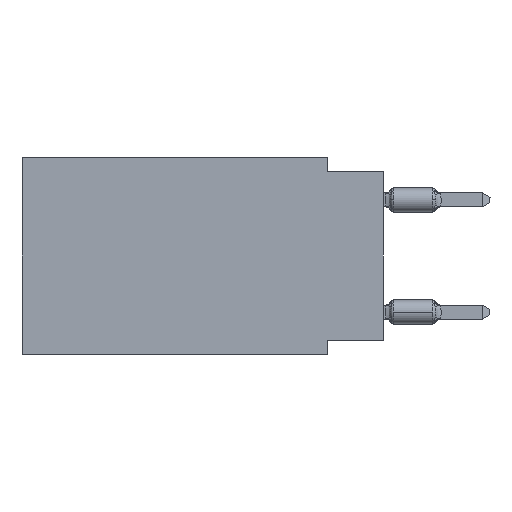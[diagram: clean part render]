
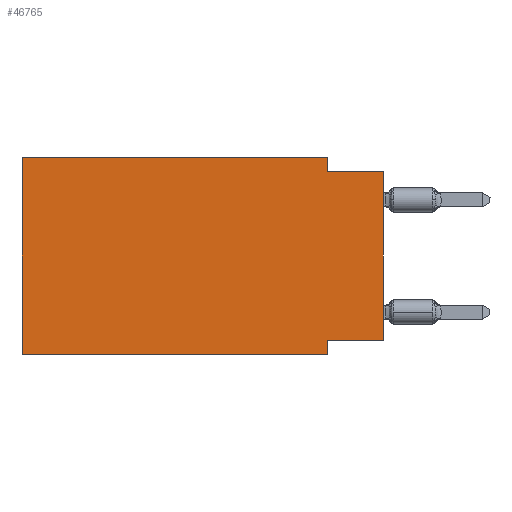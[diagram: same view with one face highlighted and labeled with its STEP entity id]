
A CAD part, left-side view. The second image highlights one B-rep face of the part: STEP entity #46765.
In plain terms, the highlighted planar face has unit normal (-1, 0, 0).
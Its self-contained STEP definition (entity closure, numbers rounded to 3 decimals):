
#680 = CARTESIAN_POINT ( 'NONE',  ( 0., 0., -8.255 ) ) ;
#1125 = EDGE_CURVE ( 'NONE', #8151, #5050, #22016, .T. ) ;
#1750 = LINE ( 'NONE', #14236, #53486 ) ;
#1891 = CARTESIAN_POINT ( 'NONE',  ( 0., 2.54, -8.255 ) ) ;
#3690 = CARTESIAN_POINT ( 'NONE',  ( 0., 2.54, -8.89 ) ) ;
#4180 = ORIENTED_EDGE ( 'NONE', *, *, #1125, .T. ) ;
#5050 = VERTEX_POINT ( 'NONE', #16949 ) ;
#5253 = DIRECTION ( 'NONE',  ( 0., -1., 0. ) ) ;
#7419 = PLANE ( 'NONE',  #43557 ) ;
#8151 = VERTEX_POINT ( 'NONE', #37151 ) ;
#10588 = VECTOR ( 'NONE', #20522, 1000. ) ;
#11175 = DIRECTION ( 'NONE',  ( 0., 0., -1. ) ) ;
#12456 = VECTOR ( 'NONE', #52749, 1000. ) ;
#13107 = VERTEX_POINT ( 'NONE', #30770 ) ;
#13301 = VECTOR ( 'NONE', #11175, 1000. ) ;
#13368 = ORIENTED_EDGE ( 'NONE', *, *, #31567, .F. ) ;
#14236 = CARTESIAN_POINT ( 'NONE',  ( 0., 0., -0.635 ) ) ;
#14434 = VECTOR ( 'NONE', #21892, 1000. ) ;
#15368 = EDGE_CURVE ( 'NONE', #13107, #5050, #1750, .T. ) ;
#16724 = VERTEX_POINT ( 'NONE', #43879 ) ;
#16949 = CARTESIAN_POINT ( 'NONE',  ( 0., 0., -0.635 ) ) ;
#19416 = EDGE_CURVE ( 'NONE', #8151, #51653, #33802, .T. ) ;
#20129 = EDGE_CURVE ( 'NONE', #25563, #13107, #27487, .T. ) ;
#20522 = DIRECTION ( 'NONE',  ( 0., 1., 0. ) ) ;
#21892 = DIRECTION ( 'NONE',  ( 0., -1., 0. ) ) ;
#22016 = LINE ( 'NONE', #34785, #38747 ) ;
#24004 = CARTESIAN_POINT ( 'NONE',  ( 0., 16.383, 0. ) ) ;
#24983 = ORIENTED_EDGE ( 'NONE', *, *, #49805, .T. ) ;
#25563 = VERTEX_POINT ( 'NONE', #28155 ) ;
#25857 = VERTEX_POINT ( 'NONE', #33251 ) ;
#25971 = CARTESIAN_POINT ( 'NONE',  ( 0., 16.383, 0. ) ) ;
#27487 = LINE ( 'NONE', #32343, #13301 ) ;
#28155 = CARTESIAN_POINT ( 'NONE',  ( 0., 2.54, 0. ) ) ;
#28202 = LINE ( 'NONE', #32821, #12456 ) ;
#30053 = LINE ( 'NONE', #25971, #14434 ) ;
#30770 = CARTESIAN_POINT ( 'NONE',  ( 0., 2.54, -0.635 ) ) ;
#31567 = EDGE_CURVE ( 'NONE', #45171, #25857, #28202, .T. ) ;
#32343 = CARTESIAN_POINT ( 'NONE',  ( 0., 2.54, 0. ) ) ;
#32821 = CARTESIAN_POINT ( 'NONE',  ( 0., 16.383, 0. ) ) ;
#32971 = CARTESIAN_POINT ( 'NONE',  ( 0., 16.383, -8.89 ) ) ;
#33251 = CARTESIAN_POINT ( 'NONE',  ( 0., 16.383, 0. ) ) ;
#33802 = LINE ( 'NONE', #680, #10588 ) ;
#34785 = CARTESIAN_POINT ( 'NONE',  ( 0., 0., 0. ) ) ;
#35544 = EDGE_LOOP ( 'NONE', ( #4180, #50564, #44331, #44738, #13368, #24983, #44711, #45854 ) ) ;
#37151 = CARTESIAN_POINT ( 'NONE',  ( 0., 0., -8.255 ) ) ;
#38606 = DIRECTION ( 'NONE',  ( 0., 0., 1. ) ) ;
#38747 = VECTOR ( 'NONE', #38606, 1000. ) ;
#39290 = EDGE_CURVE ( 'NONE', #25857, #25563, #30053, .T. ) ;
#40349 = VECTOR ( 'NONE', #40612, 1000. ) ;
#40612 = DIRECTION ( 'NONE',  ( 0., -1., 0. ) ) ;
#43557 = AXIS2_PLACEMENT_3D ( 'NONE', #24004, #43586, #47649 ) ;
#43586 = DIRECTION ( 'NONE',  ( 1., 0., 0. ) ) ;
#43879 = CARTESIAN_POINT ( 'NONE',  ( 0., 2.54, -8.89 ) ) ;
#44331 = ORIENTED_EDGE ( 'NONE', *, *, #20129, .F. ) ;
#44655 = FACE_OUTER_BOUND ( 'NONE', #35544, .T. ) ;
#44711 = ORIENTED_EDGE ( 'NONE', *, *, #48972, .F. ) ;
#44738 = ORIENTED_EDGE ( 'NONE', *, *, #39290, .F. ) ;
#45003 = LINE ( 'NONE', #3690, #48039 ) ;
#45171 = VERTEX_POINT ( 'NONE', #32971 ) ;
#45854 = ORIENTED_EDGE ( 'NONE', *, *, #19416, .F. ) ;
#46765 = ADVANCED_FACE ( 'NONE', ( #44655 ), #7419, .F. ) ;
#47649 = DIRECTION ( 'NONE',  ( 0., 0., -1. ) ) ;
#48039 = VECTOR ( 'NONE', #53419, 1000. ) ;
#48972 = EDGE_CURVE ( 'NONE', #51653, #16724, #45003, .T. ) ;
#49262 = LINE ( 'NONE', #53057, #40349 ) ;
#49805 = EDGE_CURVE ( 'NONE', #45171, #16724, #49262, .T. ) ;
#50564 = ORIENTED_EDGE ( 'NONE', *, *, #15368, .F. ) ;
#51653 = VERTEX_POINT ( 'NONE', #1891 ) ;
#52749 = DIRECTION ( 'NONE',  ( 0., 0., 1. ) ) ;
#53057 = CARTESIAN_POINT ( 'NONE',  ( 0., 16.383, -8.89 ) ) ;
#53419 = DIRECTION ( 'NONE',  ( 0., 0., -1. ) ) ;
#53486 = VECTOR ( 'NONE', #5253, 1000. ) ;
